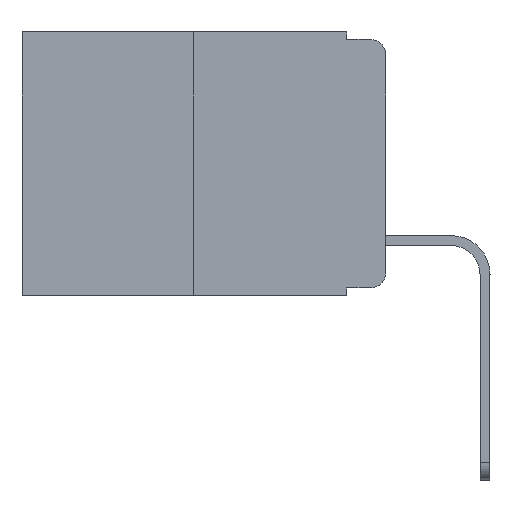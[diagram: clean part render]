
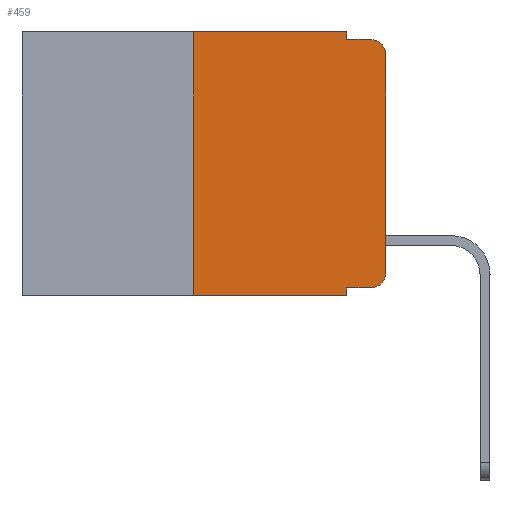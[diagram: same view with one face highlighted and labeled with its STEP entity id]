
A CAD part, left-side view. The second image highlights one B-rep face of the part: STEP entity #459.
In plain terms, the highlighted planar face has unit normal (-1, 0, 0).
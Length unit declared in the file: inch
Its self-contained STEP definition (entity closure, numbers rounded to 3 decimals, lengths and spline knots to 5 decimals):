
#58 = CARTESIAN_POINT ( 'NONE',  ( 0., 0.051, 0. ) ) ;
#459 = ADVANCED_FACE ( 'NONE', ( #760 ), #6524, .F. ) ;
#505 = LINE ( 'NONE', #616, #9586 ) ;
#616 = CARTESIAN_POINT ( 'NONE',  ( 0., 0.25, 0. ) ) ;
#760 = FACE_OUTER_BOUND ( 'NONE', #4398, .T. ) ;
#772 = ORIENTED_EDGE ( 'NONE', *, *, #9216, .T. ) ;
#840 = VECTOR ( 'NONE', #10030, 39.37008 ) ;
#1251 = EDGE_CURVE ( 'NONE', #8976, #11738, #505, .T. ) ;
#1375 = VECTOR ( 'NONE', #3098, 39.37008 ) ;
#1649 = DIRECTION ( 'NONE',  ( -1., 0., 0. ) ) ;
#1836 = CARTESIAN_POINT ( 'NONE',  ( 0., 0.051, 0. ) ) ;
#1877 = CARTESIAN_POINT ( 'NONE',  ( 0., 0.25, 0. ) ) ;
#1999 = ORIENTED_EDGE ( 'NONE', *, *, #8919, .T. ) ;
#2045 = VERTEX_POINT ( 'NONE', #7454 ) ;
#2055 = CARTESIAN_POINT ( 'NONE',  ( 0., 0.051, -0.01 ) ) ;
#2203 = CARTESIAN_POINT ( 'NONE',  ( 0., 0., 0. ) ) ;
#2295 = ORIENTED_EDGE ( 'NONE', *, *, #3645, .T. ) ;
#2654 = CARTESIAN_POINT ( 'NONE',  ( 0., 0.473, -0.343 ) ) ;
#2823 = DIRECTION ( 'NONE',  ( 0., 0., -1. ) ) ;
#2838 = ORIENTED_EDGE ( 'NONE', *, *, #14966, .F. ) ;
#2907 = CARTESIAN_POINT ( 'NONE',  ( 0., 0.02, -0.313 ) ) ;
#3052 = ORIENTED_EDGE ( 'NONE', *, *, #13072, .F. ) ;
#3098 = DIRECTION ( 'NONE',  ( 0., 0., -1. ) ) ;
#3168 = CARTESIAN_POINT ( 'NONE',  ( 0., 0.473, 0. ) ) ;
#3236 = LINE ( 'NONE', #1836, #1375 ) ;
#3248 = CARTESIAN_POINT ( 'NONE',  ( 0., 0.02, -0.01 ) ) ;
#3645 = EDGE_CURVE ( 'NONE', #10839, #9263, #8293, .T. ) ;
#3935 = VERTEX_POINT ( 'NONE', #8472 ) ;
#4398 = EDGE_LOOP ( 'NONE', ( #772, #6960, #3052, #2838, #11023, #9562, #12345, #7160, #2295, #1999 ) ) ;
#4554 = VECTOR ( 'NONE', #13731, 39.37008 ) ;
#4808 = CARTESIAN_POINT ( 'NONE',  ( 0., 0.02, -0.333 ) ) ;
#5356 = EDGE_CURVE ( 'NONE', #8976, #12003, #8706, .T. ) ;
#5392 = LINE ( 'NONE', #3168, #4554 ) ;
#5462 = EDGE_CURVE ( 'NONE', #15499, #14444, #8283, .T. ) ;
#5983 = DIRECTION ( 'NONE',  ( 0., 0., 1. ) ) ;
#6002 = VECTOR ( 'NONE', #2823, 39.37008 ) ;
#6047 = DIRECTION ( 'NONE',  ( -1., 0., 0. ) ) ;
#6353 = CARTESIAN_POINT ( 'NONE',  ( 0., 0.473, 0. ) ) ;
#6412 = AXIS2_PLACEMENT_3D ( 'NONE', #12702, #6047, #8767 ) ;
#6426 = CARTESIAN_POINT ( 'NONE',  ( 0., 0.051, -0.333 ) ) ;
#6524 = PLANE ( 'NONE',  #13859 ) ;
#6544 = DIRECTION ( 'NONE',  ( 0., -1., 0. ) ) ;
#6960 = ORIENTED_EDGE ( 'NONE', *, *, #5462, .T. ) ;
#7160 = ORIENTED_EDGE ( 'NONE', *, *, #10951, .F. ) ;
#7454 = CARTESIAN_POINT ( 'NONE',  ( 0., 0., -0.313 ) ) ;
#7460 = VECTOR ( 'NONE', #6544, 39.37008 ) ;
#7947 = VECTOR ( 'NONE', #5983, 39.37008 ) ;
#8283 = CIRCLE ( 'NONE', #6412, 0.02 ) ;
#8293 = LINE ( 'NONE', #6426, #16695 ) ;
#8472 = CARTESIAN_POINT ( 'NONE',  ( 0., 0.051, 0. ) ) ;
#8701 = LINE ( 'NONE', #2055, #840 ) ;
#8706 = LINE ( 'NONE', #2654, #7460 ) ;
#8767 = DIRECTION ( 'NONE',  ( 0., 0., -1. ) ) ;
#8919 = EDGE_CURVE ( 'NONE', #9263, #2045, #13719, .T. ) ;
#8976 = VERTEX_POINT ( 'NONE', #11961 ) ;
#9080 = DIRECTION ( 'NONE',  ( 0., -1., 0. ) ) ;
#9094 = LINE ( 'NONE', #58, #6002 ) ;
#9216 = EDGE_CURVE ( 'NONE', #2045, #15499, #9583, .T. ) ;
#9263 = VERTEX_POINT ( 'NONE', #4808 ) ;
#9562 = ORIENTED_EDGE ( 'NONE', *, *, #1251, .F. ) ;
#9583 = LINE ( 'NONE', #2203, #7947 ) ;
#9586 = VECTOR ( 'NONE', #13871, 39.37008 ) ;
#10030 = DIRECTION ( 'NONE',  ( 0., -1., 0. ) ) ;
#10414 = AXIS2_PLACEMENT_3D ( 'NONE', #2907, #1649, #15917 ) ;
#10839 = VERTEX_POINT ( 'NONE', #15769 ) ;
#10951 = EDGE_CURVE ( 'NONE', #10839, #12003, #9094, .T. ) ;
#11023 = ORIENTED_EDGE ( 'NONE', *, *, #11091, .F. ) ;
#11091 = EDGE_CURVE ( 'NONE', #11738, #3935, #5392, .T. ) ;
#11704 = DIRECTION ( 'NONE',  ( 1., 0., 0. ) ) ;
#11738 = VERTEX_POINT ( 'NONE', #1877 ) ;
#11961 = CARTESIAN_POINT ( 'NONE',  ( 0., 0.25, -0.343 ) ) ;
#12003 = VERTEX_POINT ( 'NONE', #13046 ) ;
#12345 = ORIENTED_EDGE ( 'NONE', *, *, #5356, .T. ) ;
#12702 = CARTESIAN_POINT ( 'NONE',  ( 0., 0.02, -0.03 ) ) ;
#13046 = CARTESIAN_POINT ( 'NONE',  ( 0., 0.051, -0.343 ) ) ;
#13072 = EDGE_CURVE ( 'NONE', #15727, #14444, #8701, .T. ) ;
#13402 = CARTESIAN_POINT ( 'NONE',  ( 0., 0., -0.03 ) ) ;
#13719 = CIRCLE ( 'NONE', #10414, 0.02 ) ;
#13731 = DIRECTION ( 'NONE',  ( 0., -1., 0. ) ) ;
#13761 = CARTESIAN_POINT ( 'NONE',  ( 0., 0.051, -0.01 ) ) ;
#13859 = AXIS2_PLACEMENT_3D ( 'NONE', #6353, #11704, #16953 ) ;
#13871 = DIRECTION ( 'NONE',  ( 0., 0., 1. ) ) ;
#14444 = VERTEX_POINT ( 'NONE', #3248 ) ;
#14966 = EDGE_CURVE ( 'NONE', #3935, #15727, #3236, .T. ) ;
#15499 = VERTEX_POINT ( 'NONE', #13402 ) ;
#15727 = VERTEX_POINT ( 'NONE', #13761 ) ;
#15769 = CARTESIAN_POINT ( 'NONE',  ( 0., 0.051, -0.333 ) ) ;
#15917 = DIRECTION ( 'NONE',  ( 0., 0., -1. ) ) ;
#16695 = VECTOR ( 'NONE', #9080, 39.37008 ) ;
#16953 = DIRECTION ( 'NONE',  ( 0., 0., -1. ) ) ;
